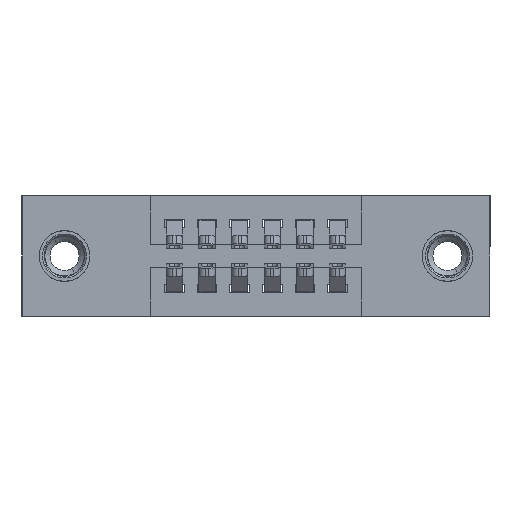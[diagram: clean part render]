
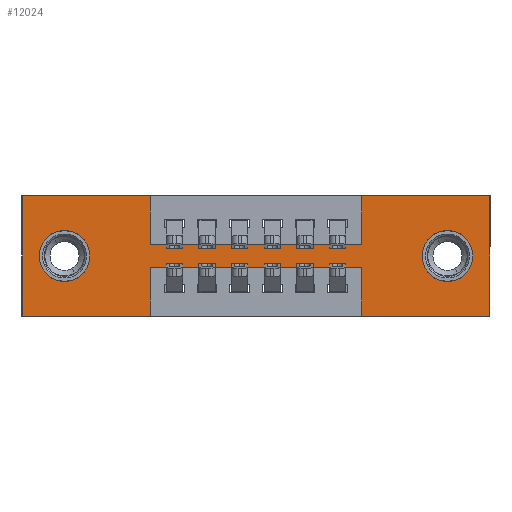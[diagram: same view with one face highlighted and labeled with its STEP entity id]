
A CAD part, front view. The second image highlights one B-rep face of the part: STEP entity #12024.
In plain terms, the highlighted planar face has unit normal (0, -1, 0).
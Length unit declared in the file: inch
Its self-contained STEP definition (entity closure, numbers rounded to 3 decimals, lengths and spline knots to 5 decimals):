
#57 = EDGE_CURVE ( 'NONE', #3966, #7503, #2360, .T. ) ;
#237 = EDGE_LOOP ( 'NONE', ( #5307, #2100, #2370, #10963, #9519, #3496, #1384, #4709, #8486, #7582, #9935, #8719 ) ) ;
#319 = DIRECTION ( 'NONE',  ( 0., 0., 1. ) ) ;
#577 = VERTEX_POINT ( 'NONE', #11521 ) ;
#606 = ORIENTED_EDGE ( 'NONE', *, *, #7562, .T. ) ;
#754 = CARTESIAN_POINT ( 'NONE',  ( 1.0425, 0., -0.37 ) ) ;
#815 = LINE ( 'NONE', #2763, #3140 ) ;
#882 = LINE ( 'NONE', #11248, #1452 ) ;
#959 = EDGE_CURVE ( 'NONE', #5576, #9504, #10695, .T. ) ;
#976 = CARTESIAN_POINT ( 'NONE',  ( 1.0425, 0., 0. ) ) ;
#1384 = ORIENTED_EDGE ( 'NONE', *, *, #2781, .F. ) ;
#1405 = ORIENTED_EDGE ( 'NONE', *, *, #8050, .T. ) ;
#1452 = VECTOR ( 'NONE', #11793, 39.37008 ) ;
#1514 = CIRCLE ( 'NONE', #8171, 0.078 ) ;
#1528 = CARTESIAN_POINT ( 'NONE',  ( 0.13, 0., -0.185 ) ) ;
#1623 = CARTESIAN_POINT ( 'NONE',  ( 1.305, 0., -0.185 ) ) ;
#1739 = VECTOR ( 'NONE', #5194, 39.37008 ) ;
#1864 = CARTESIAN_POINT ( 'NONE',  ( 1.305, 0., -0.263 ) ) ;
#2100 = ORIENTED_EDGE ( 'NONE', *, *, #5975, .F. ) ;
#2180 = FACE_BOUND ( 'NONE', #11492, .T. ) ;
#2317 = LINE ( 'NONE', #11996, #11828 ) ;
#2360 = LINE ( 'NONE', #4234, #8054 ) ;
#2370 = ORIENTED_EDGE ( 'NONE', *, *, #3879, .F. ) ;
#2452 = CARTESIAN_POINT ( 'NONE',  ( 1.435, 0., 0. ) ) ;
#2463 = CARTESIAN_POINT ( 'NONE',  ( 0., 0., 0. ) ) ;
#2522 = VERTEX_POINT ( 'NONE', #3117 ) ;
#2549 = VECTOR ( 'NONE', #5621, 39.37008 ) ;
#2560 = CARTESIAN_POINT ( 'NONE',  ( 0.3925, 0., -0.15 ) ) ;
#2586 = DIRECTION ( 'NONE',  ( -1., 0., 0. ) ) ;
#2647 = VERTEX_POINT ( 'NONE', #3147 ) ;
#2763 = CARTESIAN_POINT ( 'NONE',  ( 0., 0., 0. ) ) ;
#2781 = EDGE_CURVE ( 'NONE', #7144, #4115, #8926, .T. ) ;
#3022 = EDGE_CURVE ( 'NONE', #2647, #2522, #2317, .T. ) ;
#3117 = CARTESIAN_POINT ( 'NONE',  ( 0., 0., 0. ) ) ;
#3140 = VECTOR ( 'NONE', #9381, 39.37008 ) ;
#3147 = CARTESIAN_POINT ( 'NONE',  ( 0., 0., -0.37 ) ) ;
#3219 = CARTESIAN_POINT ( 'NONE',  ( 0.3925, 0., -0.15 ) ) ;
#3314 = DIRECTION ( 'NONE',  ( 0., 0., 1. ) ) ;
#3322 = CARTESIAN_POINT ( 'NONE',  ( 0.13, 0., -0.107 ) ) ;
#3349 = LINE ( 'NONE', #7316, #8012 ) ;
#3496 = ORIENTED_EDGE ( 'NONE', *, *, #5707, .F. ) ;
#3500 = VERTEX_POINT ( 'NONE', #5086 ) ;
#3581 = CARTESIAN_POINT ( 'NONE',  ( 0.3925, 0., -0.37 ) ) ;
#3597 = DIRECTION ( 'NONE',  ( 0., 0., -1. ) ) ;
#3601 = EDGE_CURVE ( 'NONE', #7804, #6924, #3349, .T. ) ;
#3639 = VECTOR ( 'NONE', #319, 39.37008 ) ;
#3745 = CARTESIAN_POINT ( 'NONE',  ( 0.3925, 0., -0.22 ) ) ;
#3879 = EDGE_CURVE ( 'NONE', #6924, #7504, #9473, .T. ) ;
#3966 = VERTEX_POINT ( 'NONE', #9064 ) ;
#4115 = VERTEX_POINT ( 'NONE', #976 ) ;
#4234 = CARTESIAN_POINT ( 'NONE',  ( 0.3925, 0., -0.37 ) ) ;
#4320 = CIRCLE ( 'NONE', #4930, 0.078 ) ;
#4460 = DIRECTION ( 'NONE',  ( 0., 0., 1. ) ) ;
#4516 = CARTESIAN_POINT ( 'NONE',  ( 1.0425, 0., -0.22 ) ) ;
#4709 = ORIENTED_EDGE ( 'NONE', *, *, #8663, .F. ) ;
#4723 = LINE ( 'NONE', #3745, #2549 ) ;
#4764 = CIRCLE ( 'NONE', #5320, 0.078 ) ;
#4930 = AXIS2_PLACEMENT_3D ( 'NONE', #9017, #9095, #6287 ) ;
#5080 = CARTESIAN_POINT ( 'NONE',  ( 1.0425, 0., 0. ) ) ;
#5082 = PLANE ( 'NONE',  #10345 ) ;
#5086 = CARTESIAN_POINT ( 'NONE',  ( 1.305, 0., -0.107 ) ) ;
#5114 = DIRECTION ( 'NONE',  ( 0., 0., -1. ) ) ;
#5146 = DIRECTION ( 'NONE',  ( 0., 0., -1. ) ) ;
#5194 = DIRECTION ( 'NONE',  ( 1., 0., 0. ) ) ;
#5307 = ORIENTED_EDGE ( 'NONE', *, *, #57, .F. ) ;
#5320 = AXIS2_PLACEMENT_3D ( 'NONE', #1623, #10734, #5146 ) ;
#5576 = VERTEX_POINT ( 'NONE', #6901 ) ;
#5621 = DIRECTION ( 'NONE',  ( -1., 0., 0. ) ) ;
#5707 = EDGE_CURVE ( 'NONE', #4115, #6938, #815, .T. ) ;
#5942 = DIRECTION ( 'NONE',  ( 0., -1., 0. ) ) ;
#5975 = EDGE_CURVE ( 'NONE', #7504, #3966, #4723, .T. ) ;
#5979 = CARTESIAN_POINT ( 'NONE',  ( 1.0425, 0., -0.15 ) ) ;
#6028 = DIRECTION ( 'NONE',  ( 0., 0., 1. ) ) ;
#6170 = ORIENTED_EDGE ( 'NONE', *, *, #9076, .T. ) ;
#6287 = DIRECTION ( 'NONE',  ( 0., 0., -1. ) ) ;
#6360 = LINE ( 'NONE', #2560, #10591 ) ;
#6506 = AXIS2_PLACEMENT_3D ( 'NONE', #1528, #11717, #9005 ) ;
#6680 = CARTESIAN_POINT ( 'NONE',  ( 0., 0., -0.37 ) ) ;
#6796 = EDGE_CURVE ( 'NONE', #6938, #7804, #882, .T. ) ;
#6901 = CARTESIAN_POINT ( 'NONE',  ( 0.3925, 0., 0. ) ) ;
#6924 = VERTEX_POINT ( 'NONE', #754 ) ;
#6938 = VERTEX_POINT ( 'NONE', #2452 ) ;
#6975 = DIRECTION ( 'NONE',  ( 0., 0., -1. ) ) ;
#7144 = VERTEX_POINT ( 'NONE', #5979 ) ;
#7316 = CARTESIAN_POINT ( 'NONE',  ( 0., 0., -0.37 ) ) ;
#7424 = EDGE_CURVE ( 'NONE', #2522, #5576, #8445, .T. ) ;
#7503 = VERTEX_POINT ( 'NONE', #3581 ) ;
#7504 = VERTEX_POINT ( 'NONE', #4516 ) ;
#7562 = EDGE_CURVE ( 'NONE', #10420, #3500, #4764, .T. ) ;
#7582 = ORIENTED_EDGE ( 'NONE', *, *, #7424, .F. ) ;
#7804 = VERTEX_POINT ( 'NONE', #11851 ) ;
#8012 = VECTOR ( 'NONE', #2586, 39.37008 ) ;
#8050 = EDGE_CURVE ( 'NONE', #577, #8984, #10601, .T. ) ;
#8054 = VECTOR ( 'NONE', #5114, 39.37008 ) ;
#8171 = AXIS2_PLACEMENT_3D ( 'NONE', #11673, #9807, #3314 ) ;
#8247 = EDGE_LOOP ( 'NONE', ( #8949, #1405 ) ) ;
#8445 = LINE ( 'NONE', #2463, #1739 ) ;
#8486 = ORIENTED_EDGE ( 'NONE', *, *, #959, .F. ) ;
#8521 = DIRECTION ( 'NONE',  ( -1., 0., 0. ) ) ;
#8611 = FACE_BOUND ( 'NONE', #8247, .T. ) ;
#8663 = EDGE_CURVE ( 'NONE', #9504, #7144, #6360, .T. ) ;
#8719 = ORIENTED_EDGE ( 'NONE', *, *, #11495, .F. ) ;
#8768 = CARTESIAN_POINT ( 'NONE',  ( 1.0425, 0., -0.37 ) ) ;
#8773 = VECTOR ( 'NONE', #6028, 39.37008 ) ;
#8926 = LINE ( 'NONE', #5080, #8773 ) ;
#8949 = ORIENTED_EDGE ( 'NONE', *, *, #10729, .T. ) ;
#8984 = VERTEX_POINT ( 'NONE', #3322 ) ;
#9005 = DIRECTION ( 'NONE',  ( 0., 0., 1. ) ) ;
#9017 = CARTESIAN_POINT ( 'NONE',  ( 1.305, 0., -0.185 ) ) ;
#9064 = CARTESIAN_POINT ( 'NONE',  ( 0.3925, 0., -0.22 ) ) ;
#9076 = EDGE_CURVE ( 'NONE', #3500, #10420, #4320, .T. ) ;
#9095 = DIRECTION ( 'NONE',  ( 0., 1., 0. ) ) ;
#9196 = CARTESIAN_POINT ( 'NONE',  ( 0.3925, 0., 0. ) ) ;
#9368 = VECTOR ( 'NONE', #8521, 39.37008 ) ;
#9381 = DIRECTION ( 'NONE',  ( 1., 0., 0. ) ) ;
#9473 = LINE ( 'NONE', #8768, #3639 ) ;
#9501 = LINE ( 'NONE', #6680, #9368 ) ;
#9504 = VERTEX_POINT ( 'NONE', #3219 ) ;
#9519 = ORIENTED_EDGE ( 'NONE', *, *, #6796, .F. ) ;
#9807 = DIRECTION ( 'NONE',  ( 0., 1., 0. ) ) ;
#9935 = ORIENTED_EDGE ( 'NONE', *, *, #3022, .F. ) ;
#10345 = AXIS2_PLACEMENT_3D ( 'NONE', #10645, #5942, #6975 ) ;
#10420 = VERTEX_POINT ( 'NONE', #1864 ) ;
#10591 = VECTOR ( 'NONE', #11949, 39.37008 ) ;
#10601 = CIRCLE ( 'NONE', #6506, 0.078 ) ;
#10645 = CARTESIAN_POINT ( 'NONE',  ( 0., 0., -0.37 ) ) ;
#10695 = LINE ( 'NONE', #9196, #11872 ) ;
#10729 = EDGE_CURVE ( 'NONE', #8984, #577, #1514, .T. ) ;
#10734 = DIRECTION ( 'NONE',  ( 0., 1., 0. ) ) ;
#10796 = FACE_OUTER_BOUND ( 'NONE', #237, .T. ) ;
#10963 = ORIENTED_EDGE ( 'NONE', *, *, #3601, .F. ) ;
#11248 = CARTESIAN_POINT ( 'NONE',  ( 1.435, 0., 0. ) ) ;
#11492 = EDGE_LOOP ( 'NONE', ( #6170, #606 ) ) ;
#11495 = EDGE_CURVE ( 'NONE', #7503, #2647, #9501, .T. ) ;
#11521 = CARTESIAN_POINT ( 'NONE',  ( 0.13, 0., -0.263 ) ) ;
#11673 = CARTESIAN_POINT ( 'NONE',  ( 0.13, 0., -0.185 ) ) ;
#11717 = DIRECTION ( 'NONE',  ( 0., 1., 0. ) ) ;
#11793 = DIRECTION ( 'NONE',  ( 0., 0., -1. ) ) ;
#11828 = VECTOR ( 'NONE', #4460, 39.37008 ) ;
#11851 = CARTESIAN_POINT ( 'NONE',  ( 1.435, 0., -0.37 ) ) ;
#11872 = VECTOR ( 'NONE', #3597, 39.37008 ) ;
#11949 = DIRECTION ( 'NONE',  ( 1., 0., 0. ) ) ;
#11996 = CARTESIAN_POINT ( 'NONE',  ( 0., 0., 0. ) ) ;
#12024 = ADVANCED_FACE ( 'NONE', ( #2180, #8611, #10796 ), #5082, .T. ) ;
